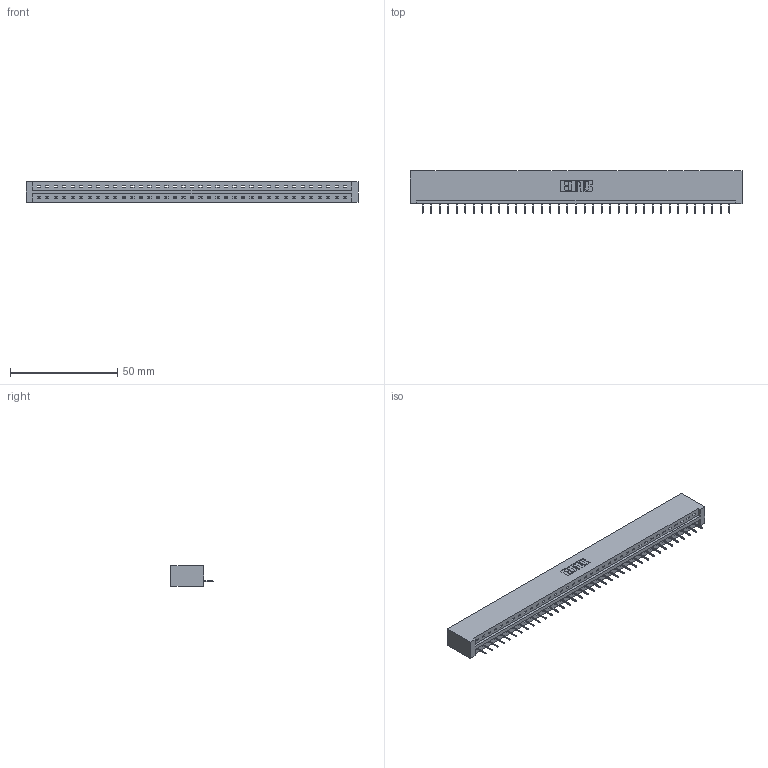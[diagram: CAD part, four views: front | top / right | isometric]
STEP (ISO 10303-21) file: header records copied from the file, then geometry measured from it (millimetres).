
FILE_DESCRIPTION (( 'STEP AP203' ), '1' );
FILE_NAME ('387-037-524-101.STEP', '2019-10-04T14:26:34', ( '' ), ( '' ), 'SwSTEP 2.0', 'SolidWorks 2016', '' );
FILE_SCHEMA (( 'CONFIG_CONTROL_DESIGN' ));
Length unit declared in the file: inch
Products named in the file (3): 345-292-001_345-293-124; 337 Part_No Mounting Lugs; 387-037-524-101
Assembly tree (38 placements, depth 2):
  387-037-524-101
    337 Part_No Mounting Lugs
    345-292-001_345-293-124  x37
Bounding box: 154.48 x 19.69 x 9.4 mm (x, y, z)
Volume: 16585.9 mm3; surface area: 16578.7 mm2
Topology: 38 solids, 38 shells, 2548 faces, 7391 edges, 4778 vertices
Faces by surface type: plane 1990, cylinder 558
Entity records: 27947 total; most frequent: CARTESIAN_POINT 4873, ORIENTED_EDGE 4846, DIRECTION 4105, EDGE_CURVE 2423, VECTOR 2307, LINE 2307, VERTEX_POINT 1610, AXIS2_PLACEMENT_3D 899
